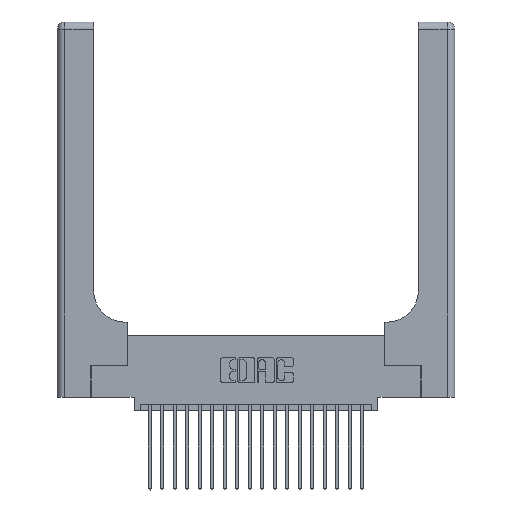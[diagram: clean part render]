
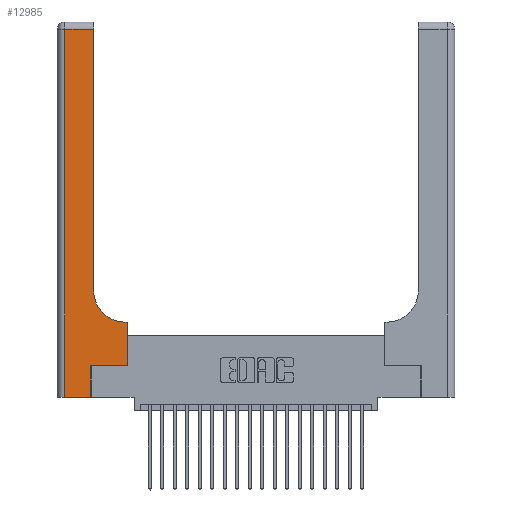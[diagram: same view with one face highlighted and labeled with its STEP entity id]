
A CAD part, top view. The second image highlights one B-rep face of the part: STEP entity #12985.
In plain terms, the highlighted planar face has unit normal (0, 0, 1).
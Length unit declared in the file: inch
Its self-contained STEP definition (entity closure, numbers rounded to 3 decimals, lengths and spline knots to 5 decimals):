
#6 = VECTOR ( 'NONE', #3369, 39.37008 ) ;
#376 = VECTOR ( 'NONE', #4642, 39.37008 ) ;
#745 = DIRECTION ( 'NONE',  ( 0., 0., -1. ) ) ;
#906 = VERTEX_POINT ( 'NONE', #5577 ) ;
#1517 = CARTESIAN_POINT ( 'NONE',  ( 0.269, 0.25, 0.37 ) ) ;
#1795 = EDGE_CURVE ( 'NONE', #12796, #9407, #5782, .T. ) ;
#1815 = CARTESIAN_POINT ( 'NONE',  ( 0.5585, 0.25, 0.37 ) ) ;
#2030 = LINE ( 'NONE', #2912, #14393 ) ;
#2483 = CARTESIAN_POINT ( 'NONE',  ( 0.2915, 3., 0.37 ) ) ;
#2566 = CARTESIAN_POINT ( 'NONE',  ( 0.269, 0., 0.37 ) ) ;
#2912 = CARTESIAN_POINT ( 'NONE',  ( 0., 2.94, 0.37 ) ) ;
#3369 = DIRECTION ( 'NONE',  ( 1., 0., 0. ) ) ;
#3612 = AXIS2_PLACEMENT_3D ( 'NONE', #16381, #745, #22229 ) ;
#3846 = ORIENTED_EDGE ( 'NONE', *, *, #15717, .T. ) ;
#4026 = EDGE_CURVE ( 'NONE', #14868, #906, #19898, .T. ) ;
#4147 = PLANE ( 'NONE',  #3612 ) ;
#4461 = EDGE_CURVE ( 'NONE', #906, #20275, #15572, .T. ) ;
#4642 = DIRECTION ( 'NONE',  ( 1., 0., 0. ) ) ;
#4693 = DIRECTION ( 'NONE',  ( 0., 0., -1. ) ) ;
#5388 = VECTOR ( 'NONE', #11399, 39.37008 ) ;
#5427 = DIRECTION ( 'NONE',  ( -1., 0., 0. ) ) ;
#5490 = CARTESIAN_POINT ( 'NONE',  ( 0.06, 0., 0.37 ) ) ;
#5577 = CARTESIAN_POINT ( 'NONE',  ( 0.5585, 0.6, 0.37 ) ) ;
#5782 = LINE ( 'NONE', #15701, #6 ) ;
#6047 = DIRECTION ( 'NONE',  ( 0., 1., 0. ) ) ;
#6213 = VECTOR ( 'NONE', #14999, 39.37008 ) ;
#6239 = EDGE_CURVE ( 'NONE', #21071, #15168, #2030, .T. ) ;
#6408 = CARTESIAN_POINT ( 'NONE',  ( 0.269, 0.25, 0.37 ) ) ;
#6824 = ORIENTED_EDGE ( 'NONE', *, *, #6239, .T. ) ;
#7004 = ORIENTED_EDGE ( 'NONE', *, *, #4026, .T. ) ;
#7510 = DIRECTION ( 'NONE',  ( 0., -1., 0. ) ) ;
#8116 = DIRECTION ( 'NONE',  ( 1., 0., 0. ) ) ;
#8224 = VECTOR ( 'NONE', #6047, 39.37008 ) ;
#9303 = CARTESIAN_POINT ( 'NONE',  ( 0.5415, 0.6, 0.37 ) ) ;
#9345 = LINE ( 'NONE', #2566, #8224 ) ;
#9407 = VERTEX_POINT ( 'NONE', #18546 ) ;
#9515 = AXIS2_PLACEMENT_3D ( 'NONE', #11602, #4693, #8116 ) ;
#9699 = ORIENTED_EDGE ( 'NONE', *, *, #18383, .T. ) ;
#10271 = ORIENTED_EDGE ( 'NONE', *, *, #1795, .T. ) ;
#10555 = EDGE_CURVE ( 'NONE', #9407, #14793, #9345, .T. ) ;
#10896 = VECTOR ( 'NONE', #5427, 39.37008 ) ;
#11153 = FACE_OUTER_BOUND ( 'NONE', #14896, .T. ) ;
#11399 = DIRECTION ( 'NONE',  ( 0., 1., 0. ) ) ;
#11602 = CARTESIAN_POINT ( 'NONE',  ( 0.5415, 0.85, 0.37 ) ) ;
#11787 = CIRCLE ( 'NONE', #9515, 0.25 ) ;
#12609 = ORIENTED_EDGE ( 'NONE', *, *, #10555, .T. ) ;
#12796 = VERTEX_POINT ( 'NONE', #5490 ) ;
#12985 = ADVANCED_FACE ( 'NONE', ( #11153 ), #4147, .F. ) ;
#13034 = LINE ( 'NONE', #6408, #376 ) ;
#13639 = CARTESIAN_POINT ( 'NONE',  ( 0.06, 2.94, 0.37 ) ) ;
#14393 = VECTOR ( 'NONE', #20126, 39.37008 ) ;
#14515 = LINE ( 'NONE', #21666, #18584 ) ;
#14793 = VERTEX_POINT ( 'NONE', #1517 ) ;
#14868 = VERTEX_POINT ( 'NONE', #1815 ) ;
#14896 = EDGE_LOOP ( 'NONE', ( #22288, #6824, #3846, #10271, #12609, #9699, #7004, #16386, #16443 ) ) ;
#14958 = LINE ( 'NONE', #2483, #5388 ) ;
#14999 = DIRECTION ( 'NONE',  ( 0., 1., 0. ) ) ;
#15168 = VERTEX_POINT ( 'NONE', #13639 ) ;
#15572 = LINE ( 'NONE', #19111, #10896 ) ;
#15701 = CARTESIAN_POINT ( 'NONE',  ( 0., 0., 0.37 ) ) ;
#15717 = EDGE_CURVE ( 'NONE', #15168, #12796, #14515, .T. ) ;
#15820 = EDGE_CURVE ( 'NONE', #20275, #20222, #11787, .T. ) ;
#16381 = CARTESIAN_POINT ( 'NONE',  ( 0., 3., 0.37 ) ) ;
#16386 = ORIENTED_EDGE ( 'NONE', *, *, #4461, .T. ) ;
#16443 = ORIENTED_EDGE ( 'NONE', *, *, #15820, .T. ) ;
#16632 = CARTESIAN_POINT ( 'NONE',  ( 0.2915, 0.85, 0.37 ) ) ;
#18383 = EDGE_CURVE ( 'NONE', #14793, #14868, #13034, .T. ) ;
#18546 = CARTESIAN_POINT ( 'NONE',  ( 0.269, 0., 0.37 ) ) ;
#18584 = VECTOR ( 'NONE', #7510, 39.37008 ) ;
#19111 = CARTESIAN_POINT ( 'NONE',  ( 0.2915, 0.6, 0.37 ) ) ;
#19898 = LINE ( 'NONE', #22430, #6213 ) ;
#20126 = DIRECTION ( 'NONE',  ( -1., 0., 0. ) ) ;
#20222 = VERTEX_POINT ( 'NONE', #16632 ) ;
#20275 = VERTEX_POINT ( 'NONE', #9303 ) ;
#21071 = VERTEX_POINT ( 'NONE', #22187 ) ;
#21341 = EDGE_CURVE ( 'NONE', #20222, #21071, #14958, .T. ) ;
#21666 = CARTESIAN_POINT ( 'NONE',  ( 0.06, 3., 0.37 ) ) ;
#22187 = CARTESIAN_POINT ( 'NONE',  ( 0.2915, 2.94, 0.37 ) ) ;
#22229 = DIRECTION ( 'NONE',  ( -1., 0., 0. ) ) ;
#22288 = ORIENTED_EDGE ( 'NONE', *, *, #21341, .T. ) ;
#22430 = CARTESIAN_POINT ( 'NONE',  ( 0.5585, 0.25, 0.37 ) ) ;
